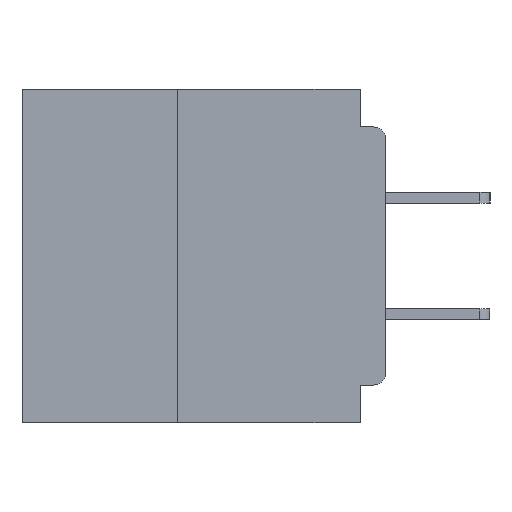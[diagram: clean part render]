
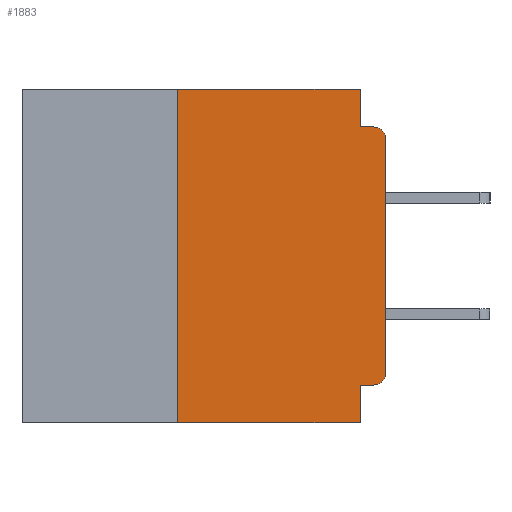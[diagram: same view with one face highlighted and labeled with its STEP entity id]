
A CAD part, left-side view. The second image highlights one B-rep face of the part: STEP entity #1883.
In plain terms, the highlighted planar face has unit normal (-1, 0, 0).
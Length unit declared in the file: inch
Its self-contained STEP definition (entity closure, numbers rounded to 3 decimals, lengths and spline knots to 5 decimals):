
#1108 = VERTEX_POINT ( 'NONE', #45114 ) ;
#1255 = CARTESIAN_POINT ( 'NONE',  ( 0., 0.031, -0.4 ) ) ;
#1883 = ADVANCED_FACE ( 'NONE', ( #47303 ), #13433, .F. ) ;
#3014 = VECTOR ( 'NONE', #37973, 39.37008 ) ;
#4510 = EDGE_CURVE ( 'NONE', #34202, #1108, #27567, .T. ) ;
#5108 = VERTEX_POINT ( 'NONE', #21683 ) ;
#5723 = DIRECTION ( 'NONE',  ( 0., 0., -1. ) ) ;
#5792 = EDGE_LOOP ( 'NONE', ( #14181, #7638, #21484, #20355, #14723, #50929, #54073, #16557, #25739, #33027 ) ) ;
#6403 = EDGE_CURVE ( 'NONE', #1108, #16189, #16215, .T. ) ;
#6992 = CARTESIAN_POINT ( 'NONE',  ( 0., 0.015, -0.34 ) ) ;
#7131 = CARTESIAN_POINT ( 'NONE',  ( 0., 0.015, -0.06 ) ) ;
#7159 = CARTESIAN_POINT ( 'NONE',  ( 0., 0.031, 0. ) ) ;
#7355 = AXIS2_PLACEMENT_3D ( 'NONE', #7131, #38139, #11607 ) ;
#7365 = CARTESIAN_POINT ( 'NONE',  ( 0., 0.437, -0.4 ) ) ;
#7638 = ORIENTED_EDGE ( 'NONE', *, *, #27847, .T. ) ;
#8873 = VECTOR ( 'NONE', #53276, 39.37008 ) ;
#11454 = DIRECTION ( 'NONE',  ( 0., 0., -1. ) ) ;
#11607 = DIRECTION ( 'NONE',  ( 0., 0., -1. ) ) ;
#11831 = DIRECTION ( 'NONE',  ( 0., -1., 0. ) ) ;
#13114 = DIRECTION ( 'NONE',  ( 0., 0., -1. ) ) ;
#13122 = DIRECTION ( 'NONE',  ( 1., 0., 0. ) ) ;
#13318 = CARTESIAN_POINT ( 'NONE',  ( 0., 0.437, 0. ) ) ;
#13433 = PLANE ( 'NONE',  #50511 ) ;
#13903 = CARTESIAN_POINT ( 'NONE',  ( 0., 0.015, -0.355 ) ) ;
#14181 = ORIENTED_EDGE ( 'NONE', *, *, #38295, .T. ) ;
#14723 = ORIENTED_EDGE ( 'NONE', *, *, #4510, .F. ) ;
#14855 = DIRECTION ( 'NONE',  ( 0., 1., 0. ) ) ;
#15104 = LINE ( 'NONE', #40259, #38666 ) ;
#16189 = VERTEX_POINT ( 'NONE', #50002 ) ;
#16215 = LINE ( 'NONE', #7159, #3014 ) ;
#16557 = ORIENTED_EDGE ( 'NONE', *, *, #20528, .F. ) ;
#16710 = VERTEX_POINT ( 'NONE', #13903 ) ;
#17818 = CARTESIAN_POINT ( 'NONE',  ( 0., 0., -0.045 ) ) ;
#18448 = VECTOR ( 'NONE', #42454, 39.37008 ) ;
#18723 = VECTOR ( 'NONE', #5723, 39.37008 ) ;
#19669 = VERTEX_POINT ( 'NONE', #48467 ) ;
#20326 = CARTESIAN_POINT ( 'NONE',  ( 0., 0.25, -0.4 ) ) ;
#20355 = ORIENTED_EDGE ( 'NONE', *, *, #6403, .F. ) ;
#20528 = EDGE_CURVE ( 'NONE', #40684, #5108, #42305, .T. ) ;
#21484 = ORIENTED_EDGE ( 'NONE', *, *, #52008, .F. ) ;
#21683 = CARTESIAN_POINT ( 'NONE',  ( 0., 0.031, -0.4 ) ) ;
#25415 = VECTOR ( 'NONE', #14855, 39.37008 ) ;
#25423 = CARTESIAN_POINT ( 'NONE',  ( 0., 0.25, 0. ) ) ;
#25739 = ORIENTED_EDGE ( 'NONE', *, *, #26497, .F. ) ;
#26497 = EDGE_CURVE ( 'NONE', #16710, #40684, #48990, .T. ) ;
#27335 = EDGE_CURVE ( 'NONE', #16710, #36030, #31672, .T. ) ;
#27567 = LINE ( 'NONE', #39964, #28967 ) ;
#27847 = EDGE_CURVE ( 'NONE', #35377, #19669, #42045, .T. ) ;
#28967 = VECTOR ( 'NONE', #31053, 39.37008 ) ;
#31001 = CARTESIAN_POINT ( 'NONE',  ( 0., 0.25, -0.4 ) ) ;
#31053 = DIRECTION ( 'NONE',  ( 0., -1., 0. ) ) ;
#31672 = CIRCLE ( 'NONE', #52299, 0.015 ) ;
#32529 = CARTESIAN_POINT ( 'NONE',  ( 0., 0.031, -0.355 ) ) ;
#33027 = ORIENTED_EDGE ( 'NONE', *, *, #27335, .T. ) ;
#34202 = VERTEX_POINT ( 'NONE', #25423 ) ;
#35377 = VERTEX_POINT ( 'NONE', #38541 ) ;
#36030 = VERTEX_POINT ( 'NONE', #55929 ) ;
#37189 = LINE ( 'NONE', #7365, #47607 ) ;
#37973 = DIRECTION ( 'NONE',  ( 0., 0., -1. ) ) ;
#37995 = DIRECTION ( 'NONE',  ( -1., 0., 0. ) ) ;
#38139 = DIRECTION ( 'NONE',  ( -1., 0., 0. ) ) ;
#38295 = EDGE_CURVE ( 'NONE', #36030, #35377, #15104, .T. ) ;
#38541 = CARTESIAN_POINT ( 'NONE',  ( 0., 0., -0.06 ) ) ;
#38666 = VECTOR ( 'NONE', #49154, 39.37008 ) ;
#39964 = CARTESIAN_POINT ( 'NONE',  ( 0., 0.437, 0. ) ) ;
#40259 = CARTESIAN_POINT ( 'NONE',  ( 0., 0., 0. ) ) ;
#40684 = VERTEX_POINT ( 'NONE', #32529 ) ;
#41442 = CARTESIAN_POINT ( 'NONE',  ( 0., 0., -0.355 ) ) ;
#42045 = CIRCLE ( 'NONE', #7355, 0.015 ) ;
#42305 = LINE ( 'NONE', #1255, #18723 ) ;
#42454 = DIRECTION ( 'NONE',  ( 0., 0., 1. ) ) ;
#43810 = EDGE_CURVE ( 'NONE', #45962, #5108, #37189, .T. ) ;
#44407 = EDGE_CURVE ( 'NONE', #45962, #34202, #52387, .T. ) ;
#45114 = CARTESIAN_POINT ( 'NONE',  ( 0., 0.031, 0. ) ) ;
#45962 = VERTEX_POINT ( 'NONE', #31001 ) ;
#47303 = FACE_OUTER_BOUND ( 'NONE', #5792, .T. ) ;
#47607 = VECTOR ( 'NONE', #11831, 39.37008 ) ;
#48467 = CARTESIAN_POINT ( 'NONE',  ( 0., 0.015, -0.045 ) ) ;
#48990 = LINE ( 'NONE', #41442, #25415 ) ;
#49154 = DIRECTION ( 'NONE',  ( 0., 0., 1. ) ) ;
#50002 = CARTESIAN_POINT ( 'NONE',  ( 0., 0.031, -0.045 ) ) ;
#50511 = AXIS2_PLACEMENT_3D ( 'NONE', #13318, #13122, #13114 ) ;
#50929 = ORIENTED_EDGE ( 'NONE', *, *, #44407, .F. ) ;
#52008 = EDGE_CURVE ( 'NONE', #16189, #19669, #55236, .T. ) ;
#52299 = AXIS2_PLACEMENT_3D ( 'NONE', #6992, #37995, #11454 ) ;
#52387 = LINE ( 'NONE', #20326, #18448 ) ;
#53276 = DIRECTION ( 'NONE',  ( 0., -1., 0. ) ) ;
#54073 = ORIENTED_EDGE ( 'NONE', *, *, #43810, .T. ) ;
#55236 = LINE ( 'NONE', #17818, #8873 ) ;
#55929 = CARTESIAN_POINT ( 'NONE',  ( 0., 0., -0.34 ) ) ;
